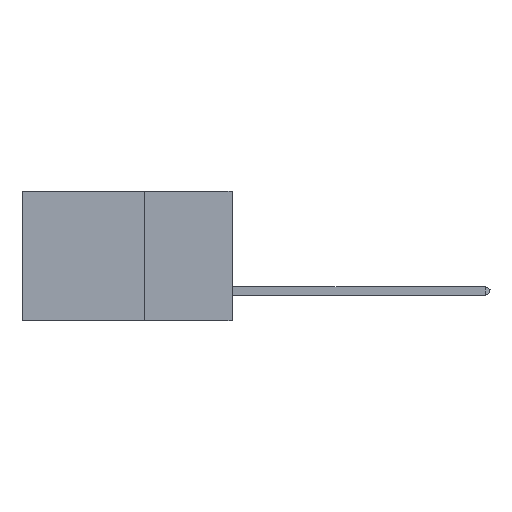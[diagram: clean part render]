
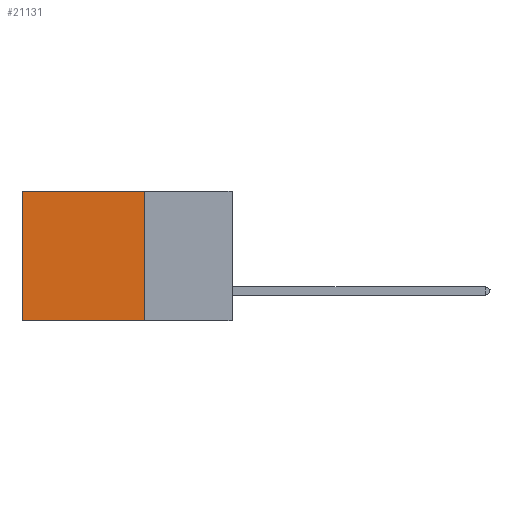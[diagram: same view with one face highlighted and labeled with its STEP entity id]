
A CAD part, left-side view. The second image highlights one B-rep face of the part: STEP entity #21131.
In plain terms, the highlighted planar face has unit normal (-1, 0, 0).
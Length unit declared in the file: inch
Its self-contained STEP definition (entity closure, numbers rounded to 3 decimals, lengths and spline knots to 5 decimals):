
#1268 = CARTESIAN_POINT ( 'NONE',  ( 0.2875, 0.25, -0.37 ) ) ;
#1559 = DIRECTION ( 'NONE',  ( 0., 0., -1. ) ) ;
#1905 = CARTESIAN_POINT ( 'NONE',  ( 0.2875, 0.25, 0. ) ) ;
#2725 = FACE_OUTER_BOUND ( 'NONE', #8052, .T. ) ;
#3682 = AXIS2_PLACEMENT_3D ( 'NONE', #33214, #6876, #23040 ) ;
#3879 = CARTESIAN_POINT ( 'NONE',  ( 0.2875, 0.25, -0.37 ) ) ;
#4446 = EDGE_CURVE ( 'NONE', #15576, #17801, #27142, .T. ) ;
#5279 = CARTESIAN_POINT ( 'NONE',  ( 0.2875, 0.6, -0.37 ) ) ;
#5410 = ORIENTED_EDGE ( 'NONE', *, *, #15882, .F. ) ;
#5639 = ORIENTED_EDGE ( 'NONE', *, *, #33845, .T. ) ;
#6876 = DIRECTION ( 'NONE',  ( 1., 0., 0. ) ) ;
#8052 = EDGE_LOOP ( 'NONE', ( #5639, #5410, #10101, #29331 ) ) ;
#8311 = VERTEX_POINT ( 'NONE', #1268 ) ;
#8559 = VERTEX_POINT ( 'NONE', #5279 ) ;
#9142 = DIRECTION ( 'NONE',  ( 0., 1., 0. ) ) ;
#10101 = ORIENTED_EDGE ( 'NONE', *, *, #11800, .F. ) ;
#10555 = LINE ( 'NONE', #3879, #16684 ) ;
#11800 = EDGE_CURVE ( 'NONE', #15576, #8311, #15681, .T. ) ;
#15576 = VERTEX_POINT ( 'NONE', #29422 ) ;
#15681 = LINE ( 'NONE', #1905, #31680 ) ;
#15882 = EDGE_CURVE ( 'NONE', #8311, #8559, #10555, .T. ) ;
#16487 = CARTESIAN_POINT ( 'NONE',  ( 0.2875, 0.6, 0. ) ) ;
#16684 = VECTOR ( 'NONE', #9142, 39.37008 ) ;
#17729 = VECTOR ( 'NONE', #31753, 39.37008 ) ;
#17801 = VERTEX_POINT ( 'NONE', #16487 ) ;
#19767 = CARTESIAN_POINT ( 'NONE',  ( 0.2875, 0.6, 0. ) ) ;
#19880 = DIRECTION ( 'NONE',  ( 0., 0., -1. ) ) ;
#21131 = ADVANCED_FACE ( 'NONE', ( #2725 ), #25572, .F. ) ;
#23040 = DIRECTION ( 'NONE',  ( 0., 0., -1. ) ) ;
#24272 = LINE ( 'NONE', #19767, #28770 ) ;
#25572 = PLANE ( 'NONE',  #3682 ) ;
#26471 = CARTESIAN_POINT ( 'NONE',  ( 0.2875, 0.25, 0. ) ) ;
#27142 = LINE ( 'NONE', #26471, #17729 ) ;
#28770 = VECTOR ( 'NONE', #19880, 39.37008 ) ;
#29331 = ORIENTED_EDGE ( 'NONE', *, *, #4446, .T. ) ;
#29422 = CARTESIAN_POINT ( 'NONE',  ( 0.2875, 0.25, 0. ) ) ;
#31680 = VECTOR ( 'NONE', #1559, 39.37008 ) ;
#31753 = DIRECTION ( 'NONE',  ( 0., 1., 0. ) ) ;
#33214 = CARTESIAN_POINT ( 'NONE',  ( 0.2875, 0.25, 0. ) ) ;
#33845 = EDGE_CURVE ( 'NONE', #17801, #8559, #24272, .T. ) ;
